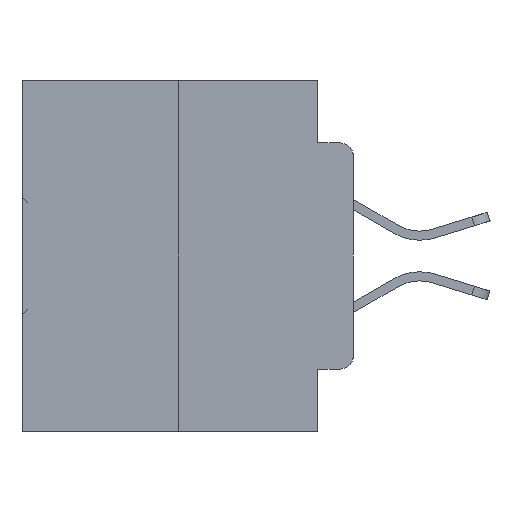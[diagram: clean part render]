
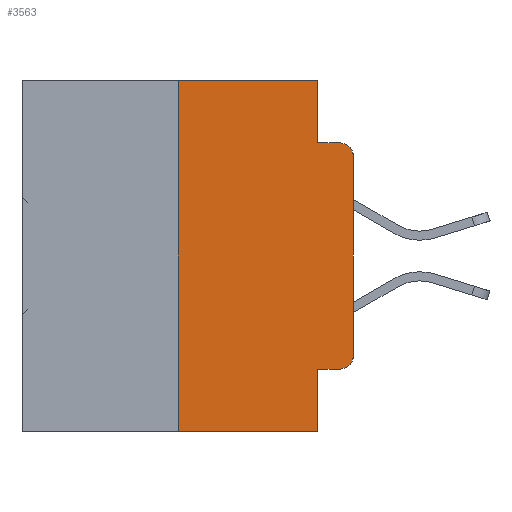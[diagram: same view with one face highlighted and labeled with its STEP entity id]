
A CAD part, left-side view. The second image highlights one B-rep face of the part: STEP entity #3563.
In plain terms, the highlighted planar face has unit normal (-1, 0, 0).
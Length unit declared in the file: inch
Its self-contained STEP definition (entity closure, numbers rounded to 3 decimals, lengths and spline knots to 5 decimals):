
#19 = CARTESIAN_POINT ( 'NONE',  ( 0., 0.051, -0.5 ) ) ;
#99 = VERTEX_POINT ( 'NONE', #12788 ) ;
#1460 = AXIS2_PLACEMENT_3D ( 'NONE', #20663, #31834, #31712 ) ;
#2277 = DIRECTION ( 'NONE',  ( 0., 0., -1. ) ) ;
#2897 = AXIS2_PLACEMENT_3D ( 'NONE', #30749, #15173, #33317 ) ;
#3563 = ADVANCED_FACE ( 'NONE', ( #25164 ), #24167, .F. ) ;
#3984 = VERTEX_POINT ( 'NONE', #23853 ) ;
#4128 = CARTESIAN_POINT ( 'NONE',  ( 0., 0.25, -0.5 ) ) ;
#4598 = EDGE_CURVE ( 'NONE', #5565, #21906, #4911, .T. ) ;
#4911 = CIRCLE ( 'NONE', #30819, 0.02 ) ;
#5565 = VERTEX_POINT ( 'NONE', #24181 ) ;
#5729 = VERTEX_POINT ( 'NONE', #26402 ) ;
#7746 = DIRECTION ( 'NONE',  ( 0., -1., 0. ) ) ;
#8823 = EDGE_LOOP ( 'NONE', ( #23337, #23107, #13584, #33274, #28090, #25089, #11958, #8939, #10875, #16300 ) ) ;
#8882 = VERTEX_POINT ( 'NONE', #22660 ) ;
#8939 = ORIENTED_EDGE ( 'NONE', *, *, #24234, .F. ) ;
#9018 = VERTEX_POINT ( 'NONE', #4128 ) ;
#9952 = LINE ( 'NONE', #25154, #30790 ) ;
#10491 = EDGE_CURVE ( 'NONE', #9018, #11470, #9952, .T. ) ;
#10810 = LINE ( 'NONE', #17960, #29204 ) ;
#10875 = ORIENTED_EDGE ( 'NONE', *, *, #18991, .T. ) ;
#11172 = VECTOR ( 'NONE', #7746, 39.37008 ) ;
#11229 = CARTESIAN_POINT ( 'NONE',  ( 0., 0.051, 0. ) ) ;
#11247 = CARTESIAN_POINT ( 'NONE',  ( 0., 0.051, 0. ) ) ;
#11470 = VERTEX_POINT ( 'NONE', #19 ) ;
#11958 = ORIENTED_EDGE ( 'NONE', *, *, #10491, .T. ) ;
#12308 = LINE ( 'NONE', #14991, #33032 ) ;
#12547 = LINE ( 'NONE', #15356, #24011 ) ;
#12788 = CARTESIAN_POINT ( 'NONE',  ( 0., 0., -0.3915 ) ) ;
#13584 = ORIENTED_EDGE ( 'NONE', *, *, #21165, .F. ) ;
#13911 = DIRECTION ( 'NONE',  ( 0., 0., -1. ) ) ;
#14991 = CARTESIAN_POINT ( 'NONE',  ( 0., 0.051, -0.0885 ) ) ;
#15173 = DIRECTION ( 'NONE',  ( -1., 0., 0. ) ) ;
#15356 = CARTESIAN_POINT ( 'NONE',  ( 0., 0., 0. ) ) ;
#15851 = CIRCLE ( 'NONE', #2897, 0.02 ) ;
#16300 = ORIENTED_EDGE ( 'NONE', *, *, #33496, .T. ) ;
#16322 = LINE ( 'NONE', #11229, #20808 ) ;
#16931 = VECTOR ( 'NONE', #21902, 39.37008 ) ;
#17028 = EDGE_CURVE ( 'NONE', #99, #5565, #12547, .T. ) ;
#17960 = CARTESIAN_POINT ( 'NONE',  ( 0., 0.25, 0. ) ) ;
#18008 = DIRECTION ( 'NONE',  ( 0., 0., 1. ) ) ;
#18160 = VECTOR ( 'NONE', #19037, 39.37008 ) ;
#18176 = LINE ( 'NONE', #26028, #11172 ) ;
#18258 = CARTESIAN_POINT ( 'NONE',  ( 0., 0.02, -0.1085 ) ) ;
#18297 = DIRECTION ( 'NONE',  ( -1., 0., 0. ) ) ;
#18991 = EDGE_CURVE ( 'NONE', #33263, #29310, #31952, .T. ) ;
#19037 = DIRECTION ( 'NONE',  ( 0., -1., 0. ) ) ;
#20194 = CARTESIAN_POINT ( 'NONE',  ( 0., 0.02, -0.0885 ) ) ;
#20579 = DIRECTION ( 'NONE',  ( 0., 0., 1. ) ) ;
#20663 = CARTESIAN_POINT ( 'NONE',  ( 0., 0.473, 0. ) ) ;
#20808 = VECTOR ( 'NONE', #13911, 39.37008 ) ;
#21165 = EDGE_CURVE ( 'NONE', #8882, #21906, #12308, .T. ) ;
#21631 = CARTESIAN_POINT ( 'NONE',  ( 0., 0.051, -0.4115 ) ) ;
#21902 = DIRECTION ( 'NONE',  ( 0., 0., -1. ) ) ;
#21906 = VERTEX_POINT ( 'NONE', #20194 ) ;
#22660 = CARTESIAN_POINT ( 'NONE',  ( 0., 0.051, -0.0885 ) ) ;
#23107 = ORIENTED_EDGE ( 'NONE', *, *, #4598, .T. ) ;
#23337 = ORIENTED_EDGE ( 'NONE', *, *, #17028, .T. ) ;
#23853 = CARTESIAN_POINT ( 'NONE',  ( 0., 0.25, 0. ) ) ;
#24011 = VECTOR ( 'NONE', #18008, 39.37008 ) ;
#24167 = PLANE ( 'NONE',  #1460 ) ;
#24181 = CARTESIAN_POINT ( 'NONE',  ( 0., 0., -0.1085 ) ) ;
#24234 = EDGE_CURVE ( 'NONE', #33263, #11470, #16322, .T. ) ;
#24697 = CARTESIAN_POINT ( 'NONE',  ( 0., 0.051, -0.4115 ) ) ;
#25089 = ORIENTED_EDGE ( 'NONE', *, *, #27053, .F. ) ;
#25154 = CARTESIAN_POINT ( 'NONE',  ( 0., 0.473, -0.5 ) ) ;
#25164 = FACE_OUTER_BOUND ( 'NONE', #8823, .T. ) ;
#26028 = CARTESIAN_POINT ( 'NONE',  ( 0., 0.473, 0. ) ) ;
#26402 = CARTESIAN_POINT ( 'NONE',  ( 0., 0.051, 0. ) ) ;
#27053 = EDGE_CURVE ( 'NONE', #9018, #3984, #10810, .T. ) ;
#27724 = DIRECTION ( 'NONE',  ( 0., -1., 0. ) ) ;
#28090 = ORIENTED_EDGE ( 'NONE', *, *, #30234, .F. ) ;
#29204 = VECTOR ( 'NONE', #20579, 39.37008 ) ;
#29310 = VERTEX_POINT ( 'NONE', #30063 ) ;
#30063 = CARTESIAN_POINT ( 'NONE',  ( 0., 0.02, -0.4115 ) ) ;
#30234 = EDGE_CURVE ( 'NONE', #3984, #5729, #18176, .T. ) ;
#30498 = EDGE_CURVE ( 'NONE', #5729, #8882, #30732, .T. ) ;
#30732 = LINE ( 'NONE', #11247, #16931 ) ;
#30749 = CARTESIAN_POINT ( 'NONE',  ( 0., 0.02, -0.3915 ) ) ;
#30790 = VECTOR ( 'NONE', #27724, 39.37008 ) ;
#30819 = AXIS2_PLACEMENT_3D ( 'NONE', #18258, #18297, #2277 ) ;
#31712 = DIRECTION ( 'NONE',  ( 0., 0., -1. ) ) ;
#31834 = DIRECTION ( 'NONE',  ( 1., 0., 0. ) ) ;
#31952 = LINE ( 'NONE', #21631, #18160 ) ;
#33032 = VECTOR ( 'NONE', #33254, 39.37008 ) ;
#33254 = DIRECTION ( 'NONE',  ( 0., -1., 0. ) ) ;
#33263 = VERTEX_POINT ( 'NONE', #24697 ) ;
#33274 = ORIENTED_EDGE ( 'NONE', *, *, #30498, .F. ) ;
#33317 = DIRECTION ( 'NONE',  ( 0., 0., -1. ) ) ;
#33496 = EDGE_CURVE ( 'NONE', #29310, #99, #15851, .T. ) ;
